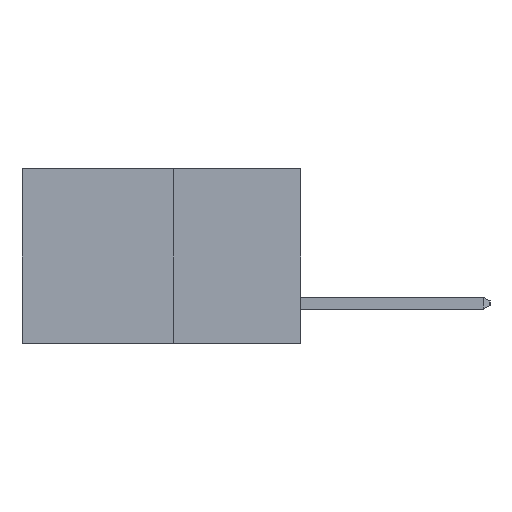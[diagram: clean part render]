
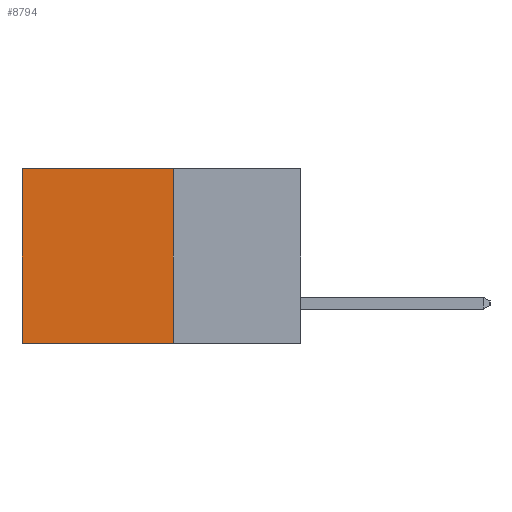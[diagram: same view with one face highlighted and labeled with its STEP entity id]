
A CAD part, left-side view. The second image highlights one B-rep face of the part: STEP entity #8794.
In plain terms, the highlighted planar face has unit normal (-1, 0, 0).
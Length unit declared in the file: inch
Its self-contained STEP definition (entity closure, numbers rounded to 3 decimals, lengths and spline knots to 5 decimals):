
#91 = DIRECTION ( 'NONE',  ( 0., 1., 0. ) ) ;
#360 = VERTEX_POINT ( 'NONE', #2321 ) ;
#676 = DIRECTION ( 'NONE',  ( 0., 0., -1. ) ) ;
#802 = VERTEX_POINT ( 'NONE', #7852 ) ;
#1027 = CARTESIAN_POINT ( 'NONE',  ( 0.277, 0.27, -0.37 ) ) ;
#1337 = VECTOR ( 'NONE', #91, 39.37008 ) ;
#1914 = LINE ( 'NONE', #9271, #6866 ) ;
#1952 = LINE ( 'NONE', #8453, #1337 ) ;
#2009 = EDGE_CURVE ( 'NONE', #802, #10977, #10534, .T. ) ;
#2321 = CARTESIAN_POINT ( 'NONE',  ( 0.277, 0.59, -0.37 ) ) ;
#3037 = CARTESIAN_POINT ( 'NONE',  ( 0.277, 0.27, -0.37 ) ) ;
#3322 = CARTESIAN_POINT ( 'NONE',  ( 0.277, 0.59, 0. ) ) ;
#3852 = DIRECTION ( 'NONE',  ( 0., 1., 0. ) ) ;
#4745 = DIRECTION ( 'NONE',  ( 0., 0., -1. ) ) ;
#4811 = ORIENTED_EDGE ( 'NONE', *, *, #2009, .F. ) ;
#4957 = VECTOR ( 'NONE', #4745, 39.37008 ) ;
#5061 = ORIENTED_EDGE ( 'NONE', *, *, #11602, .F. ) ;
#5279 = ORIENTED_EDGE ( 'NONE', *, *, #10347, .T. ) ;
#6328 = DIRECTION ( 'NONE',  ( 1., 0., 0. ) ) ;
#6866 = VECTOR ( 'NONE', #3852, 39.37008 ) ;
#7293 = AXIS2_PLACEMENT_3D ( 'NONE', #9820, #6328, #676 ) ;
#7487 = EDGE_CURVE ( 'NONE', #11291, #360, #11585, .T. ) ;
#7852 = CARTESIAN_POINT ( 'NONE',  ( 0.277, 0.27, 0. ) ) ;
#8453 = CARTESIAN_POINT ( 'NONE',  ( 0.277, 0.27, 0. ) ) ;
#8696 = ORIENTED_EDGE ( 'NONE', *, *, #7487, .T. ) ;
#8794 = ADVANCED_FACE ( 'NONE', ( #9420 ), #11598, .F. ) ;
#8982 = DIRECTION ( 'NONE',  ( 0., 0., -1. ) ) ;
#9011 = EDGE_LOOP ( 'NONE', ( #8696, #5061, #4811, #5279 ) ) ;
#9271 = CARTESIAN_POINT ( 'NONE',  ( 0.277, 0.27, -0.37 ) ) ;
#9420 = FACE_OUTER_BOUND ( 'NONE', #9011, .T. ) ;
#9811 = CARTESIAN_POINT ( 'NONE',  ( 0.277, 0.59, -0.37 ) ) ;
#9820 = CARTESIAN_POINT ( 'NONE',  ( 0.277, 0.27, -0.37 ) ) ;
#10347 = EDGE_CURVE ( 'NONE', #802, #11291, #1952, .T. ) ;
#10534 = LINE ( 'NONE', #3037, #4957 ) ;
#10977 = VERTEX_POINT ( 'NONE', #1027 ) ;
#11031 = VECTOR ( 'NONE', #8982, 39.37008 ) ;
#11291 = VERTEX_POINT ( 'NONE', #3322 ) ;
#11585 = LINE ( 'NONE', #9811, #11031 ) ;
#11598 = PLANE ( 'NONE',  #7293 ) ;
#11602 = EDGE_CURVE ( 'NONE', #10977, #360, #1914, .T. ) ;
